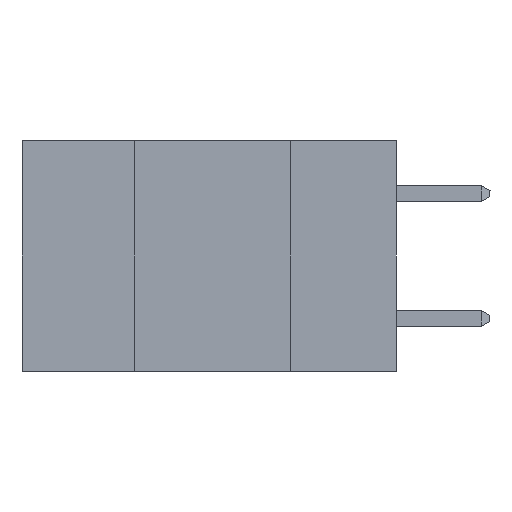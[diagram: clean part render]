
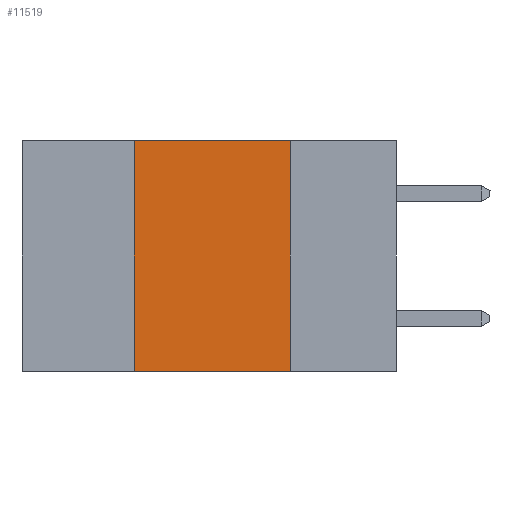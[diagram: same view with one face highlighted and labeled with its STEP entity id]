
A CAD part, left-side view. The second image highlights one B-rep face of the part: STEP entity #11519.
In plain terms, the highlighted planar face has unit normal (-1, 0, 0).
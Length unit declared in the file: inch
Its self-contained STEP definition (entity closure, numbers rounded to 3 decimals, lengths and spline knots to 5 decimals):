
#492 = LINE ( 'NONE', #23337, #4271 ) ;
#1000 = EDGE_CURVE ( 'NONE', #6164, #14563, #19800, .T. ) ;
#1742 = EDGE_CURVE ( 'NONE', #6164, #2512, #13899, .T. ) ;
#2512 = VERTEX_POINT ( 'NONE', #12187 ) ;
#3549 = DIRECTION ( 'NONE',  ( 0., -1., 0. ) ) ;
#4049 = DIRECTION ( 'NONE',  ( 0., 0., 1. ) ) ;
#4271 = VECTOR ( 'NONE', #14474, 39.37008 ) ;
#4899 = VECTOR ( 'NONE', #7028, 39.37008 ) ;
#6138 = EDGE_LOOP ( 'NONE', ( #8433, #9347, #7642, #22404 ) ) ;
#6164 = VERTEX_POINT ( 'NONE', #23118 ) ;
#7028 = DIRECTION ( 'NONE',  ( 0., 0., -1. ) ) ;
#7642 = ORIENTED_EDGE ( 'NONE', *, *, #1742, .F. ) ;
#7763 = DIRECTION ( 'NONE',  ( 1., 0., 0. ) ) ;
#8393 = CARTESIAN_POINT ( 'NONE',  ( 0., 0.42, 0. ) ) ;
#8433 = ORIENTED_EDGE ( 'NONE', *, *, #18587, .F. ) ;
#8928 = CARTESIAN_POINT ( 'NONE',  ( 0., 0.17, -0.37 ) ) ;
#9347 = ORIENTED_EDGE ( 'NONE', *, *, #22798, .F. ) ;
#9539 = CARTESIAN_POINT ( 'NONE',  ( 0., 0.6, 0. ) ) ;
#11519 = ADVANCED_FACE ( 'NONE', ( #13190 ), #16935, .F. ) ;
#12187 = CARTESIAN_POINT ( 'NONE',  ( 0., 0.42, 0. ) ) ;
#12587 = CARTESIAN_POINT ( 'NONE',  ( 0., 0.17, 0. ) ) ;
#13190 = FACE_OUTER_BOUND ( 'NONE', #6138, .T. ) ;
#13371 = AXIS2_PLACEMENT_3D ( 'NONE', #9539, #7763, #20463 ) ;
#13899 = LINE ( 'NONE', #8393, #18096 ) ;
#14178 = VERTEX_POINT ( 'NONE', #22631 ) ;
#14474 = DIRECTION ( 'NONE',  ( 0., -1., 0. ) ) ;
#14563 = VERTEX_POINT ( 'NONE', #8928 ) ;
#15593 = CARTESIAN_POINT ( 'NONE',  ( 0., 0.6, -0.37 ) ) ;
#16935 = PLANE ( 'NONE',  #13371 ) ;
#18096 = VECTOR ( 'NONE', #4049, 39.37008 ) ;
#18587 = EDGE_CURVE ( 'NONE', #14178, #14563, #23674, .T. ) ;
#19800 = LINE ( 'NONE', #15593, #23394 ) ;
#20463 = DIRECTION ( 'NONE',  ( 0., 0., -1. ) ) ;
#22404 = ORIENTED_EDGE ( 'NONE', *, *, #1000, .T. ) ;
#22631 = CARTESIAN_POINT ( 'NONE',  ( 0., 0.17, 0. ) ) ;
#22798 = EDGE_CURVE ( 'NONE', #2512, #14178, #492, .T. ) ;
#23118 = CARTESIAN_POINT ( 'NONE',  ( 0., 0.42, -0.37 ) ) ;
#23337 = CARTESIAN_POINT ( 'NONE',  ( 0., 0.6, 0. ) ) ;
#23394 = VECTOR ( 'NONE', #3549, 39.37008 ) ;
#23674 = LINE ( 'NONE', #12587, #4899 ) ;
